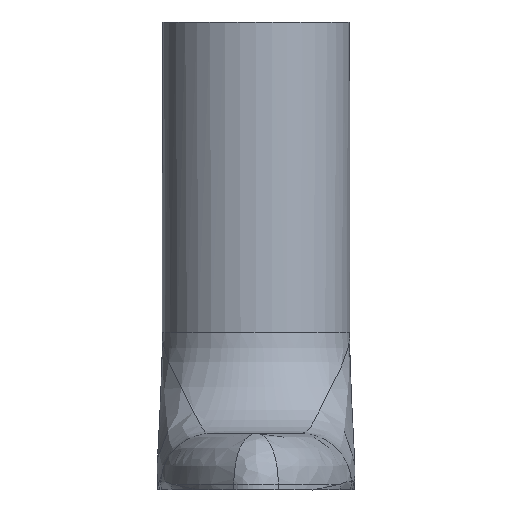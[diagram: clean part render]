
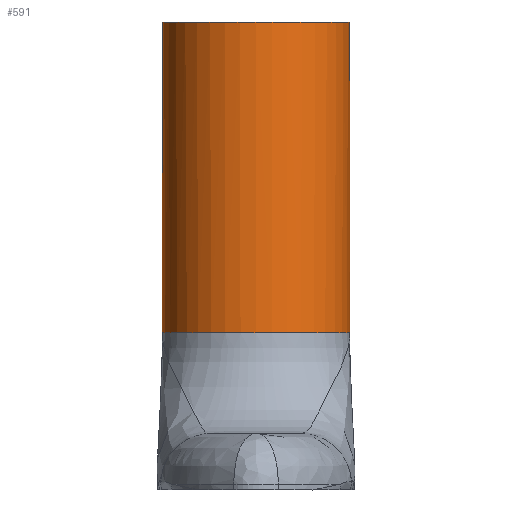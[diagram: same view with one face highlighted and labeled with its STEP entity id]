
A CAD part, front view. The second image highlights one B-rep face of the part: STEP entity #591.
In plain terms, the highlighted cylindrical face has radius 18.575 mm (diameter 37.15 mm), a partial arc.
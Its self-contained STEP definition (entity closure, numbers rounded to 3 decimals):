
#34 = CARTESIAN_POINT ( 'NONE',  ( 31.282, 62.032, 167.169 ) ) ;
#50 = DIRECTION ( 'NONE',  ( 0., 0., -1. ) ) ;
#56 = B_SPLINE_CURVE_WITH_KNOTS ( 'NONE', 3,
 ( #1317, #1474, #1132, #1126, #1122, #1107, #1102, #1094 ),
 .UNSPECIFIED., .F., .F.,
 ( 4, 2, 2, 4 ),
 ( 0., 0.001, 0.001, 0.003 ),
 .UNSPECIFIED. ) ;
#163 = ORIENTED_EDGE ( 'NONE', *, *, #1254, .T. ) ;
#173 = VECTOR ( 'NONE', #1348, 1000. ) ;
#176 = CARTESIAN_POINT ( 'NONE',  ( 12.715, 62.59, 167.169 ) ) ;
#182 = DIRECTION ( 'NONE',  ( -1., 0., 0. ) ) ;
#186 = B_SPLINE_CURVE_WITH_KNOTS ( 'NONE', 3,
 ( #1724, #854, #1711, #1689, #1659, #1571, #994, #1409, #1247, #1404 ),
 .UNSPECIFIED., .F., .F.,
 ( 4, 2, 2, 2, 4 ),
 ( 0., 0.001, 0.001, 0.002, 0.003 ),
 .UNSPECIFIED. ) ;
#188 = LINE ( 'NONE', #34, #1599 ) ;
#191 = DIRECTION ( 'NONE',  ( 0., 0., -1. ) ) ;
#196 = DIRECTION ( 'NONE',  ( 1., 0., 0. ) ) ;
#204 = DIRECTION ( 'NONE',  ( 0., 0., -1. ) ) ;
#214 = CARTESIAN_POINT ( 'NONE',  ( 12.715, 62.59, 31.866 ) ) ;
#238 = CARTESIAN_POINT ( 'NONE',  ( 31.282, 62.032, -32.094 ) ) ;
#241 = EDGE_LOOP ( 'NONE', ( #1454, #330, #1567, #1060, #1732, #163 ) ) ;
#243 = VERTEX_POINT ( 'NONE', #1179 ) ;
#253 = EDGE_CURVE ( 'NONE', #763, #348, #1604, .T. ) ;
#308 = CARTESIAN_POINT ( 'NONE',  ( 31.282, 62.032, 31.866 ) ) ;
#330 = ORIENTED_EDGE ( 'NONE', *, *, #936, .T. ) ;
#348 = VERTEX_POINT ( 'NONE', #989 ) ;
#370 = CARTESIAN_POINT ( 'NONE',  ( -5.851, 62.032, -32.094 ) ) ;
#404 = CARTESIAN_POINT ( 'NONE',  ( -5.851, 62.032, 167.169 ) ) ;
#565 = AXIS2_PLACEMENT_3D ( 'NONE', #176, #191, #182 ) ;
#580 = VERTEX_POINT ( 'NONE', #308 ) ;
#591 = ADVANCED_FACE ( 'NONE', ( #1521 ), #1167, .T. ) ;
#637 = EDGE_CURVE ( 'NONE', #913, #763, #186, .T. ) ;
#763 = VERTEX_POINT ( 'NONE', #1401 ) ;
#821 = AXIS2_PLACEMENT_3D ( 'NONE', #214, #204, #196 ) ;
#854 = CARTESIAN_POINT ( 'NONE',  ( -5.851, 62.032, -31.882 ) ) ;
#913 = VERTEX_POINT ( 'NONE', #370 ) ;
#936 = EDGE_CURVE ( 'NONE', #580, #243, #1398, .T. ) ;
#989 = CARTESIAN_POINT ( 'NONE',  ( 31.24, 61.229, -29.766 ) ) ;
#994 = CARTESIAN_POINT ( 'NONE',  ( -5.84, 61.731, -30.446 ) ) ;
#1036 = EDGE_CURVE ( 'NONE', #580, #1077, #188, .T. ) ;
#1051 = DIRECTION ( 'NONE',  ( 1., 0., 0. ) ) ;
#1055 = DIRECTION ( 'NONE',  ( 0., 0., 1. ) ) ;
#1059 = CARTESIAN_POINT ( 'NONE',  ( 12.715, 62.59, -29.766 ) ) ;
#1060 = ORIENTED_EDGE ( 'NONE', *, *, #637, .T. ) ;
#1077 = VERTEX_POINT ( 'NONE', #238 ) ;
#1094 = CARTESIAN_POINT ( 'NONE',  ( 31.282, 62.032, -32.094 ) ) ;
#1102 = CARTESIAN_POINT ( 'NONE',  ( 31.282, 62.032, -31.671 ) ) ;
#1107 = CARTESIAN_POINT ( 'NONE',  ( 31.281, 61.996, -31.252 ) ) ;
#1122 = CARTESIAN_POINT ( 'NONE',  ( 31.274, 61.813, -30.642 ) ) ;
#1126 = CARTESIAN_POINT ( 'NONE',  ( 31.271, 61.731, -30.446 ) ) ;
#1132 = CARTESIAN_POINT ( 'NONE',  ( 31.26, 61.516, -30.083 ) ) ;
#1167 = CYLINDRICAL_SURFACE ( 'NONE', #565, 18.575 ) ;
#1179 = CARTESIAN_POINT ( 'NONE',  ( -5.851, 62.032, 31.866 ) ) ;
#1209 = LINE ( 'NONE', #404, #173 ) ;
#1247 = CARTESIAN_POINT ( 'NONE',  ( -5.821, 61.38, -29.913 ) ) ;
#1254 = EDGE_CURVE ( 'NONE', #348, #1077, #56, .T. ) ;
#1317 = CARTESIAN_POINT ( 'NONE',  ( 31.24, 61.229, -29.766 ) ) ;
#1348 = DIRECTION ( 'NONE',  ( 0., 0., -1. ) ) ;
#1398 = CIRCLE ( 'NONE', #821, 18.575 ) ;
#1401 = CARTESIAN_POINT ( 'NONE',  ( -5.81, 61.229, -29.766 ) ) ;
#1404 = CARTESIAN_POINT ( 'NONE',  ( -5.81, 61.229, -29.766 ) ) ;
#1409 = CARTESIAN_POINT ( 'NONE',  ( -5.829, 61.515, -30.081 ) ) ;
#1454 = ORIENTED_EDGE ( 'NONE', *, *, #1036, .F. ) ;
#1474 = CARTESIAN_POINT ( 'NONE',  ( 31.252, 61.381, -29.915 ) ) ;
#1490 = AXIS2_PLACEMENT_3D ( 'NONE', #1059, #1055, #1051 ) ;
#1521 = FACE_OUTER_BOUND ( 'NONE', #241, .T. ) ;
#1567 = ORIENTED_EDGE ( 'NONE', *, *, #1705, .T. ) ;
#1571 = CARTESIAN_POINT ( 'NONE',  ( -5.843, 61.812, -30.64 ) ) ;
#1599 = VECTOR ( 'NONE', #50, 1000. ) ;
#1604 = CIRCLE ( 'NONE', #1490, 18.575 ) ;
#1659 = CARTESIAN_POINT ( 'NONE',  ( -5.848, 61.933, -31.043 ) ) ;
#1689 = CARTESIAN_POINT ( 'NONE',  ( -5.849, 61.973, -31.253 ) ) ;
#1705 = EDGE_CURVE ( 'NONE', #243, #913, #1209, .T. ) ;
#1711 = CARTESIAN_POINT ( 'NONE',  ( -5.851, 62.022, -31.672 ) ) ;
#1724 = CARTESIAN_POINT ( 'NONE',  ( -5.851, 62.032, -32.094 ) ) ;
#1732 = ORIENTED_EDGE ( 'NONE', *, *, #253, .T. ) ;
